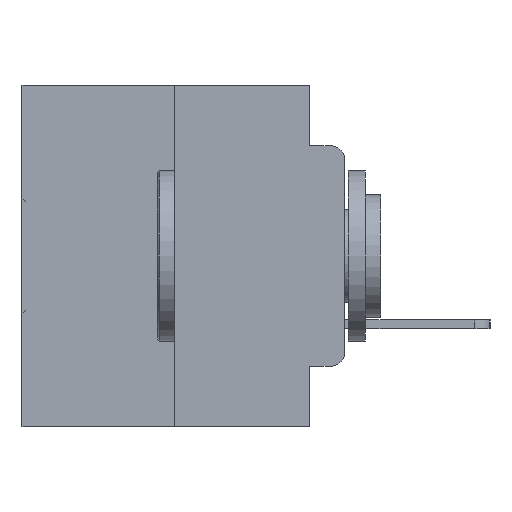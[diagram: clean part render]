
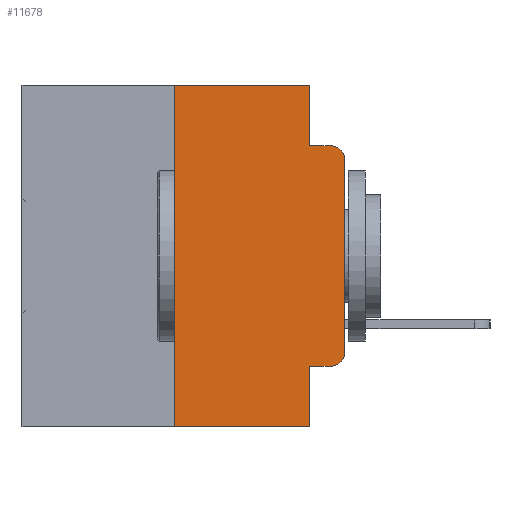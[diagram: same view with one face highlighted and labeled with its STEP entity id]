
A CAD part, left-side view. The second image highlights one B-rep face of the part: STEP entity #11678.
In plain terms, the highlighted planar face has unit normal (-1, 0, 0).
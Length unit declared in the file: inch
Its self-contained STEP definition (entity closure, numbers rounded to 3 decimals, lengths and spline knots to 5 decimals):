
#562 = CARTESIAN_POINT ( 'NONE',  ( 0., 0.25, -0.5 ) ) ;
#624 = DIRECTION ( 'NONE',  ( 0., 0., -1. ) ) ;
#720 = EDGE_CURVE ( 'NONE', #14103, #28981, #12971, .T. ) ;
#839 = ORIENTED_EDGE ( 'NONE', *, *, #28781, .F. ) ;
#1330 = PLANE ( 'NONE',  #19404 ) ;
#2022 = EDGE_CURVE ( 'NONE', #17532, #25139, #3457, .T. ) ;
#2559 = CARTESIAN_POINT ( 'NONE',  ( 0., 0.051, -0.5 ) ) ;
#2949 = DIRECTION ( 'NONE',  ( 0., -1., 0. ) ) ;
#3404 = LINE ( 'NONE', #28578, #16238 ) ;
#3457 = LINE ( 'NONE', #9960, #15514 ) ;
#3925 = EDGE_CURVE ( 'NONE', #5724, #20133, #11961, .T. ) ;
#4613 = CARTESIAN_POINT ( 'NONE',  ( 0., 0., -0.3915 ) ) ;
#5281 = CIRCLE ( 'NONE', #18713, 0.02 ) ;
#5581 = VECTOR ( 'NONE', #15424, 39.37008 ) ;
#5724 = VERTEX_POINT ( 'NONE', #19150 ) ;
#6307 = DIRECTION ( 'NONE',  ( 0., 0., -1. ) ) ;
#6571 = VECTOR ( 'NONE', #19664, 39.37008 ) ;
#6578 = VECTOR ( 'NONE', #28528, 39.37008 ) ;
#8418 = ORIENTED_EDGE ( 'NONE', *, *, #11932, .F. ) ;
#8802 = VECTOR ( 'NONE', #2949, 39.37008 ) ;
#9960 = CARTESIAN_POINT ( 'NONE',  ( 0., 0., 0. ) ) ;
#10683 = DIRECTION ( 'NONE',  ( -1., 0., 0. ) ) ;
#11033 = LINE ( 'NONE', #29049, #8802 ) ;
#11192 = CARTESIAN_POINT ( 'NONE',  ( 0., 0.051, 0. ) ) ;
#11593 = VECTOR ( 'NONE', #19655, 39.37008 ) ;
#11678 = ADVANCED_FACE ( 'NONE', ( #29193 ), #1330, .F. ) ;
#11771 = VERTEX_POINT ( 'NONE', #28099 ) ;
#11932 = EDGE_CURVE ( 'NONE', #15993, #5724, #17338, .T. ) ;
#11961 = LINE ( 'NONE', #29459, #5581 ) ;
#12971 = LINE ( 'NONE', #11192, #6571 ) ;
#12975 = LINE ( 'NONE', #19280, #6578 ) ;
#13067 = CARTESIAN_POINT ( 'NONE',  ( 0., 0.25, 0. ) ) ;
#13429 = CARTESIAN_POINT ( 'NONE',  ( 0., 0.473, 0. ) ) ;
#14044 = ORIENTED_EDGE ( 'NONE', *, *, #3925, .F. ) ;
#14103 = VERTEX_POINT ( 'NONE', #24053 ) ;
#14825 = DIRECTION ( 'NONE',  ( 0., 0., 1. ) ) ;
#15204 = DIRECTION ( 'NONE',  ( -1., 0., 0. ) ) ;
#15424 = DIRECTION ( 'NONE',  ( 0., 0., -1. ) ) ;
#15514 = VECTOR ( 'NONE', #14825, 39.37008 ) ;
#15519 = VECTOR ( 'NONE', #19136, 39.37008 ) ;
#15893 = EDGE_CURVE ( 'NONE', #27309, #28981, #11033, .T. ) ;
#15993 = VERTEX_POINT ( 'NONE', #13067 ) ;
#16014 = EDGE_CURVE ( 'NONE', #11771, #17532, #24232, .T. ) ;
#16238 = VECTOR ( 'NONE', #21703, 39.37008 ) ;
#16502 = AXIS2_PLACEMENT_3D ( 'NONE', #25068, #10683, #27348 ) ;
#17338 = LINE ( 'NONE', #26588, #11593 ) ;
#17532 = VERTEX_POINT ( 'NONE', #4613 ) ;
#17947 = ORIENTED_EDGE ( 'NONE', *, *, #27060, .T. ) ;
#18713 = AXIS2_PLACEMENT_3D ( 'NONE', #29260, #15204, #624 ) ;
#19136 = DIRECTION ( 'NONE',  ( 0., -1., 0. ) ) ;
#19150 = CARTESIAN_POINT ( 'NONE',  ( 0., 0.051, 0. ) ) ;
#19280 = CARTESIAN_POINT ( 'NONE',  ( 0., 0.051, -0.4115 ) ) ;
#19404 = AXIS2_PLACEMENT_3D ( 'NONE', #13429, #20798, #6307 ) ;
#19560 = ORIENTED_EDGE ( 'NONE', *, *, #2022, .T. ) ;
#19655 = DIRECTION ( 'NONE',  ( 0., -1., 0. ) ) ;
#19664 = DIRECTION ( 'NONE',  ( 0., 0., -1. ) ) ;
#20133 = VERTEX_POINT ( 'NONE', #25429 ) ;
#20359 = EDGE_CURVE ( 'NONE', #27309, #15993, #3404, .T. ) ;
#20549 = EDGE_CURVE ( 'NONE', #25139, #23305, #5281, .T. ) ;
#20798 = DIRECTION ( 'NONE',  ( 1., 0., 0. ) ) ;
#21005 = CARTESIAN_POINT ( 'NONE',  ( 0., 0., -0.1085 ) ) ;
#21233 = LINE ( 'NONE', #30585, #15519 ) ;
#21331 = ORIENTED_EDGE ( 'NONE', *, *, #15893, .T. ) ;
#21703 = DIRECTION ( 'NONE',  ( 0., 0., 1. ) ) ;
#23305 = VERTEX_POINT ( 'NONE', #29474 ) ;
#24053 = CARTESIAN_POINT ( 'NONE',  ( 0., 0.051, -0.4115 ) ) ;
#24232 = CIRCLE ( 'NONE', #16502, 0.02 ) ;
#25068 = CARTESIAN_POINT ( 'NONE',  ( 0., 0.02, -0.3915 ) ) ;
#25139 = VERTEX_POINT ( 'NONE', #21005 ) ;
#25429 = CARTESIAN_POINT ( 'NONE',  ( 0., 0.051, -0.0885 ) ) ;
#25702 = ORIENTED_EDGE ( 'NONE', *, *, #20549, .T. ) ;
#26588 = CARTESIAN_POINT ( 'NONE',  ( 0., 0.473, 0. ) ) ;
#27060 = EDGE_CURVE ( 'NONE', #14103, #11771, #12975, .T. ) ;
#27309 = VERTEX_POINT ( 'NONE', #562 ) ;
#27348 = DIRECTION ( 'NONE',  ( 0., 0., -1. ) ) ;
#28099 = CARTESIAN_POINT ( 'NONE',  ( 0., 0.02, -0.4115 ) ) ;
#28105 = ORIENTED_EDGE ( 'NONE', *, *, #20359, .F. ) ;
#28390 = EDGE_LOOP ( 'NONE', ( #19560, #25702, #839, #14044, #8418, #28105, #21331, #28839, #17947, #30269 ) ) ;
#28528 = DIRECTION ( 'NONE',  ( 0., -1., 0. ) ) ;
#28578 = CARTESIAN_POINT ( 'NONE',  ( 0., 0.25, 0. ) ) ;
#28781 = EDGE_CURVE ( 'NONE', #20133, #23305, #21233, .T. ) ;
#28839 = ORIENTED_EDGE ( 'NONE', *, *, #720, .F. ) ;
#28981 = VERTEX_POINT ( 'NONE', #2559 ) ;
#29049 = CARTESIAN_POINT ( 'NONE',  ( 0., 0.473, -0.5 ) ) ;
#29193 = FACE_OUTER_BOUND ( 'NONE', #28390, .T. ) ;
#29260 = CARTESIAN_POINT ( 'NONE',  ( 0., 0.02, -0.1085 ) ) ;
#29459 = CARTESIAN_POINT ( 'NONE',  ( 0., 0.051, 0. ) ) ;
#29474 = CARTESIAN_POINT ( 'NONE',  ( 0., 0.02, -0.0885 ) ) ;
#30269 = ORIENTED_EDGE ( 'NONE', *, *, #16014, .T. ) ;
#30585 = CARTESIAN_POINT ( 'NONE',  ( 0., 0.051, -0.0885 ) ) ;
